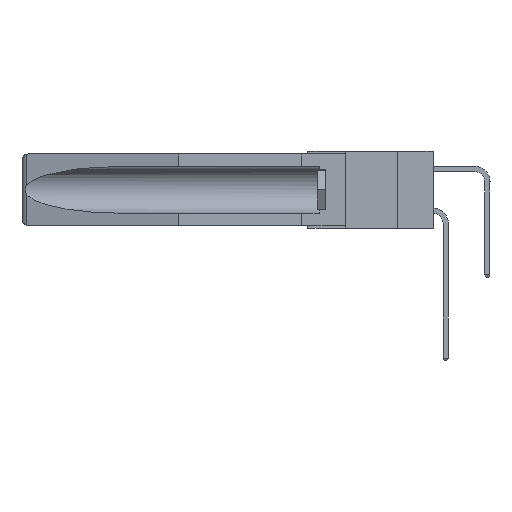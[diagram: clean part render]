
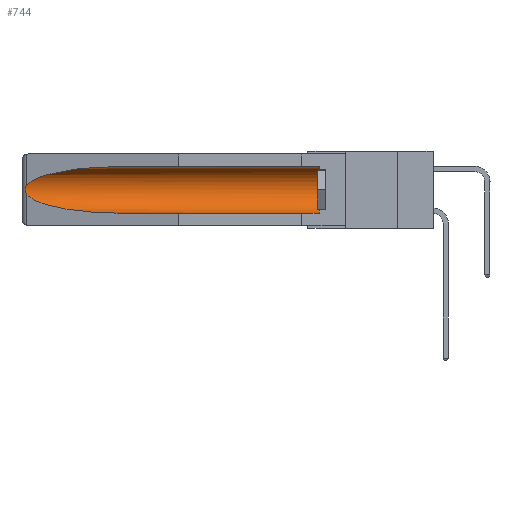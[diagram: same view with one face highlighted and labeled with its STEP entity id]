
A CAD part, left-side view. The second image highlights one B-rep face of the part: STEP entity #744.
In plain terms, the highlighted cylindrical face has radius 2.857 mm (diameter 5.715 mm), a partial arc.
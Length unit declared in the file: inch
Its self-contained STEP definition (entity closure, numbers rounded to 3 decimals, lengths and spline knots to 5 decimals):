
#698 = EDGE_CURVE ( 'NONE', #2484, #17674, #12737, .T. ) ;
#744 = ADVANCED_FACE ( 'NONE', ( #20569 ), #2317, .F. ) ;
#815 = CARTESIAN_POINT ( 'NONE',  ( 0.26655, 1.53094, -0.18657 ) ) ;
#839 = DIRECTION ( 'NONE',  ( 0., 0., 1. ) ) ;
#1407 = EDGE_CURVE ( 'NONE', #20988, #5119, #4895, .T. ) ;
#1531 = AXIS2_PLACEMENT_3D ( 'NONE', #16140, #15318, #2169 ) ;
#2169 = DIRECTION ( 'NONE',  ( 0., 0., 1. ) ) ;
#2317 = CYLINDRICAL_SURFACE ( 'NONE', #1531, 0.1125 ) ;
#2484 = VERTEX_POINT ( 'NONE', #6676 ) ;
#2700 = VERTEX_POINT ( 'NONE', #20444 ) ;
#3167 = ORIENTED_EDGE ( 'NONE', *, *, #698, .T. ) ;
#3266 = LINE ( 'NONE', #11749, #15129 ) ;
#3521 =( BOUNDED_CURVE ( )  B_SPLINE_CURVE ( 3, ( #3745, #22082, #7575, #20450 ),
 .UNSPECIFIED., .F., .F. ) 
 B_SPLINE_CURVE_WITH_KNOTS ( ( 4, 4 ),
 ( 0.1948, 1.5708 ),
 .UNSPECIFIED. ) 
 CURVE ( )  GEOMETRIC_REPRESENTATION_ITEM ( )  RATIONAL_B_SPLINE_CURVE ( ( 1., 0.848, 0.848, 1. ) ) 
 REPRESENTATION_ITEM ( '' )  );
#3745 = CARTESIAN_POINT ( 'NONE',  ( 0.26537, 1.52718, -0.19328 ) ) ;
#4124 = VECTOR ( 'NONE', #22024, 39.37008 ) ;
#4323 = DIRECTION ( 'NONE',  ( 0., -1., 0. ) ) ;
#4421 = LINE ( 'NONE', #14557, #4124 ) ;
#4554 = CARTESIAN_POINT ( 'NONE',  ( 0.2675, 1.53308, -0.16763 ) ) ;
#4895 = B_SPLINE_CURVE_WITH_KNOTS ( 'NONE', 3,
 ( #8188, #22800, #10044, #13617, #4554, #23049, #11893, #815, #13776, #19355 ),
 .UNSPECIFIED., .F., .F.,
 ( 4, 2, 2, 2, 4 ),
 ( 0., 0.00029, 0.00058, 0.00087, 0.00117 ),
 .UNSPECIFIED. ) ;
#5119 = VERTEX_POINT ( 'NONE', #20292 ) ;
#5752 = CARTESIAN_POINT ( 'NONE',  ( 0.26537, 1.52718, -0.14972 ) ) ;
#6143 = EDGE_CURVE ( 'NONE', #5119, #10560, #3521, .T. ) ;
#6676 = CARTESIAN_POINT ( 'NONE',  ( 0.155, 0.126, -0.284 ) ) ;
#6688 = EDGE_LOOP ( 'NONE', ( #9260, #17497, #14452, #16113, #3167, #22386 ) ) ;
#7575 = CARTESIAN_POINT ( 'NONE',  ( 0.21114, 1.30732, -0.284 ) ) ;
#8188 = CARTESIAN_POINT ( 'NONE',  ( 0.26537, 1.52718, -0.14972 ) ) ;
#9260 = ORIENTED_EDGE ( 'NONE', *, *, #16918, .T. ) ;
#10044 = CARTESIAN_POINT ( 'NONE',  ( 0.26654, 1.53092, -0.15636 ) ) ;
#10560 = VERTEX_POINT ( 'NONE', #16072 ) ;
#11749 = CARTESIAN_POINT ( 'NONE',  ( 0.155, -0.30754, -0.059 ) ) ;
#11893 = CARTESIAN_POINT ( 'NONE',  ( 0.2673, 1.53269, -0.17917 ) ) ;
#12159 =( BOUNDED_CURVE ( )  B_SPLINE_CURVE ( 3, ( #12658, #20332, #16446, #23965 ),
 .UNSPECIFIED., .F., .F. ) 
 B_SPLINE_CURVE_WITH_KNOTS ( ( 4, 4 ),
 ( 4.71239, 6.08839 ),
 .UNSPECIFIED. ) 
 CURVE ( )  GEOMETRIC_REPRESENTATION_ITEM ( )  RATIONAL_B_SPLINE_CURVE ( ( 1., 0.848, 0.848, 1. ) ) 
 REPRESENTATION_ITEM ( '' )  );
#12171 = CARTESIAN_POINT ( 'NONE',  ( 0.155, 0.126, -0.059 ) ) ;
#12658 = CARTESIAN_POINT ( 'NONE',  ( 0.155, 1.07973, -0.059 ) ) ;
#12737 = CIRCLE ( 'NONE', #21406, 0.1125 ) ;
#13568 = CARTESIAN_POINT ( 'NONE',  ( 0.155, 0.126, -0.1715 ) ) ;
#13617 = CARTESIAN_POINT ( 'NONE',  ( 0.2673, 1.5327, -0.16383 ) ) ;
#13776 = CARTESIAN_POINT ( 'NONE',  ( 0.26597, 1.5296, -0.19026 ) ) ;
#14452 = ORIENTED_EDGE ( 'NONE', *, *, #6143, .T. ) ;
#14557 = CARTESIAN_POINT ( 'NONE',  ( 0.155, -0.30754, -0.284 ) ) ;
#15129 = VECTOR ( 'NONE', #15472, 39.37008 ) ;
#15318 = DIRECTION ( 'NONE',  ( 0., 1., 0. ) ) ;
#15472 = DIRECTION ( 'NONE',  ( 0., 1., 0. ) ) ;
#16072 = CARTESIAN_POINT ( 'NONE',  ( 0.155, 1.07973, -0.284 ) ) ;
#16113 = ORIENTED_EDGE ( 'NONE', *, *, #21391, .F. ) ;
#16140 = CARTESIAN_POINT ( 'NONE',  ( 0.155, -0.30754, -0.1715 ) ) ;
#16446 = CARTESIAN_POINT ( 'NONE',  ( 0.25451, 1.48313, -0.09465 ) ) ;
#16918 = EDGE_CURVE ( 'NONE', #2700, #20988, #12159, .T. ) ;
#17497 = ORIENTED_EDGE ( 'NONE', *, *, #1407, .T. ) ;
#17674 = VERTEX_POINT ( 'NONE', #12171 ) ;
#19355 = CARTESIAN_POINT ( 'NONE',  ( 0.26537, 1.52718, -0.19328 ) ) ;
#20292 = CARTESIAN_POINT ( 'NONE',  ( 0.26537, 1.52718, -0.19328 ) ) ;
#20332 = CARTESIAN_POINT ( 'NONE',  ( 0.21114, 1.30732, -0.059 ) ) ;
#20444 = CARTESIAN_POINT ( 'NONE',  ( 0.155, 1.07973, -0.059 ) ) ;
#20450 = CARTESIAN_POINT ( 'NONE',  ( 0.155, 1.07973, -0.284 ) ) ;
#20569 = FACE_OUTER_BOUND ( 'NONE', #6688, .T. ) ;
#20988 = VERTEX_POINT ( 'NONE', #5752 ) ;
#21071 = EDGE_CURVE ( 'NONE', #17674, #2700, #3266, .T. ) ;
#21391 = EDGE_CURVE ( 'NONE', #2484, #10560, #4421, .T. ) ;
#21406 = AXIS2_PLACEMENT_3D ( 'NONE', #13568, #4323, #839 ) ;
#22024 = DIRECTION ( 'NONE',  ( 0., 1., 0. ) ) ;
#22082 = CARTESIAN_POINT ( 'NONE',  ( 0.25451, 1.48313, -0.24835 ) ) ;
#22386 = ORIENTED_EDGE ( 'NONE', *, *, #21071, .T. ) ;
#22800 = CARTESIAN_POINT ( 'NONE',  ( 0.26597, 1.52961, -0.15275 ) ) ;
#23049 = CARTESIAN_POINT ( 'NONE',  ( 0.2675, 1.53308, -0.17534 ) ) ;
#23965 = CARTESIAN_POINT ( 'NONE',  ( 0.26537, 1.52718, -0.14972 ) ) ;
